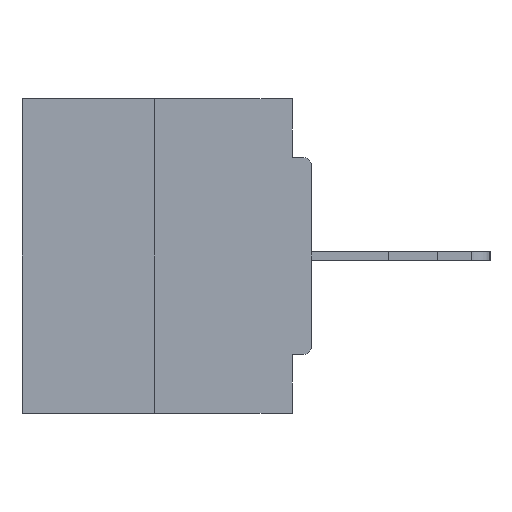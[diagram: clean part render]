
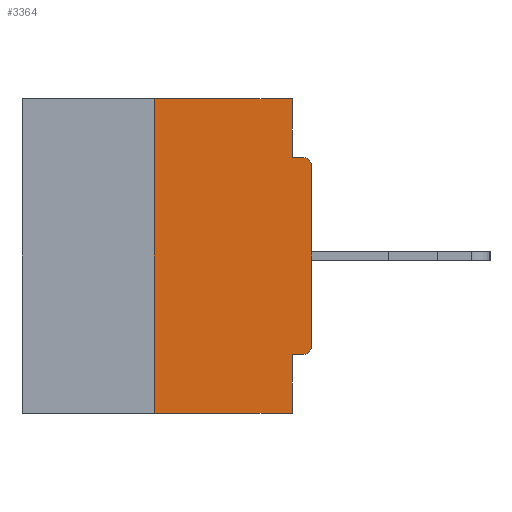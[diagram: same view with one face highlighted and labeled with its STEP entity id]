
A CAD part, left-side view. The second image highlights one B-rep face of the part: STEP entity #3364.
In plain terms, the highlighted planar face has unit normal (-1, 0, 0).
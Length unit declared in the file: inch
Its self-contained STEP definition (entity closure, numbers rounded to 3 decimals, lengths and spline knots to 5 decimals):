
#55 = FACE_OUTER_BOUND ( 'NONE', #7087, .T. ) ;
#73 = LINE ( 'NONE', #16672, #9234 ) ;
#126 = CARTESIAN_POINT ( 'NONE',  ( 0., 0.015, -0.0935 ) ) ;
#410 = CARTESIAN_POINT ( 'NONE',  ( 0., 0., -0.4065 ) ) ;
#1468 = EDGE_CURVE ( 'NONE', #32105, #14670, #10368, .T. ) ;
#2022 = CARTESIAN_POINT ( 'NONE',  ( 0., 0.015, -0.4065 ) ) ;
#3066 = EDGE_CURVE ( 'NONE', #25264, #31497, #32591, .T. ) ;
#3364 = ADVANCED_FACE ( 'NONE', ( #55 ), #19361, .F. ) ;
#3743 = LINE ( 'NONE', #22718, #32855 ) ;
#3805 = CIRCLE ( 'NONE', #9006, 0.015 ) ;
#3923 = CARTESIAN_POINT ( 'NONE',  ( 0., 0.25, 0. ) ) ;
#4043 = CARTESIAN_POINT ( 'NONE',  ( 0., 0.031, -0.4065 ) ) ;
#4228 = EDGE_CURVE ( 'NONE', #17173, #25264, #30328, .T. ) ;
#5555 = CARTESIAN_POINT ( 'NONE',  ( 0., 0.46, 0. ) ) ;
#5597 = EDGE_CURVE ( 'NONE', #6720, #14635, #3743, .T. ) ;
#5639 = CARTESIAN_POINT ( 'NONE',  ( 0., 0.031, -0.5 ) ) ;
#5778 = DIRECTION ( 'NONE',  ( -1., 0., 0. ) ) ;
#6102 = VECTOR ( 'NONE', #27866, 39.37008 ) ;
#6159 = DIRECTION ( 'NONE',  ( 0., 0., -1. ) ) ;
#6409 = EDGE_CURVE ( 'NONE', #32105, #17173, #73, .T. ) ;
#6720 = VERTEX_POINT ( 'NONE', #30334 ) ;
#7087 = EDGE_LOOP ( 'NONE', ( #32565, #34400, #19141, #24221, #24549, #12323, #35749, #17140, #16503, #34561 ) ) ;
#7121 = AXIS2_PLACEMENT_3D ( 'NONE', #14281, #5778, #6159 ) ;
#8180 = DIRECTION ( 'NONE',  ( -1., 0., 0. ) ) ;
#8782 = CARTESIAN_POINT ( 'NONE',  ( 0., 0., -0.0935 ) ) ;
#9006 = AXIS2_PLACEMENT_3D ( 'NONE', #16490, #8180, #11053 ) ;
#9234 = VECTOR ( 'NONE', #17524, 39.37008 ) ;
#10368 = LINE ( 'NONE', #29895, #19078 ) ;
#11053 = DIRECTION ( 'NONE',  ( 0., 0., -1. ) ) ;
#11419 = VECTOR ( 'NONE', #21452, 39.37008 ) ;
#11682 = DIRECTION ( 'NONE',  ( 0., 0., 1. ) ) ;
#12323 = ORIENTED_EDGE ( 'NONE', *, *, #14468, .T. ) ;
#12875 = CIRCLE ( 'NONE', #7121, 0.015 ) ;
#13216 = CARTESIAN_POINT ( 'NONE',  ( 0., 0.031, 0. ) ) ;
#14020 = LINE ( 'NONE', #8782, #33083 ) ;
#14063 = CARTESIAN_POINT ( 'NONE',  ( 0., 0.031, 0. ) ) ;
#14281 = CARTESIAN_POINT ( 'NONE',  ( 0., 0.015, -0.1085 ) ) ;
#14468 = EDGE_CURVE ( 'NONE', #30010, #6720, #3805, .T. ) ;
#14564 = EDGE_CURVE ( 'NONE', #19833, #14670, #30408, .T. ) ;
#14635 = VERTEX_POINT ( 'NONE', #25871 ) ;
#14670 = VERTEX_POINT ( 'NONE', #31123 ) ;
#15772 = EDGE_CURVE ( 'NONE', #31497, #31030, #14020, .T. ) ;
#16490 = CARTESIAN_POINT ( 'NONE',  ( 0., 0.015, -0.3915 ) ) ;
#16503 = ORIENTED_EDGE ( 'NONE', *, *, #15772, .F. ) ;
#16672 = CARTESIAN_POINT ( 'NONE',  ( 0., 0.25, 0. ) ) ;
#16907 = AXIS2_PLACEMENT_3D ( 'NONE', #30569, #19172, #24426 ) ;
#17140 = ORIENTED_EDGE ( 'NONE', *, *, #31890, .T. ) ;
#17173 = VERTEX_POINT ( 'NONE', #3923 ) ;
#17204 = CARTESIAN_POINT ( 'NONE',  ( 0., 0.031, -0.0935 ) ) ;
#17524 = DIRECTION ( 'NONE',  ( 0., 0., 1. ) ) ;
#18834 = DIRECTION ( 'NONE',  ( 0., 0., -1. ) ) ;
#19028 = DIRECTION ( 'NONE',  ( 0., -1., 0. ) ) ;
#19078 = VECTOR ( 'NONE', #19028, 39.37008 ) ;
#19141 = ORIENTED_EDGE ( 'NONE', *, *, #1468, .T. ) ;
#19172 = DIRECTION ( 'NONE',  ( 1., 0., 0. ) ) ;
#19361 = PLANE ( 'NONE',  #16907 ) ;
#19833 = VERTEX_POINT ( 'NONE', #4043 ) ;
#20471 = EDGE_CURVE ( 'NONE', #30010, #19833, #33476, .T. ) ;
#20882 = VECTOR ( 'NONE', #32403, 39.37008 ) ;
#21452 = DIRECTION ( 'NONE',  ( 0., -1., 0. ) ) ;
#22718 = CARTESIAN_POINT ( 'NONE',  ( 0., 0., 0. ) ) ;
#23989 = VECTOR ( 'NONE', #18834, 39.37008 ) ;
#24221 = ORIENTED_EDGE ( 'NONE', *, *, #14564, .F. ) ;
#24426 = DIRECTION ( 'NONE',  ( 0., 0., -1. ) ) ;
#24549 = ORIENTED_EDGE ( 'NONE', *, *, #20471, .F. ) ;
#25048 = DIRECTION ( 'NONE',  ( 0., -1., 0. ) ) ;
#25264 = VERTEX_POINT ( 'NONE', #14063 ) ;
#25871 = CARTESIAN_POINT ( 'NONE',  ( 0., 0., -0.1085 ) ) ;
#27866 = DIRECTION ( 'NONE',  ( 0., 1., 0. ) ) ;
#29895 = CARTESIAN_POINT ( 'NONE',  ( 0., 0.46, -0.5 ) ) ;
#30010 = VERTEX_POINT ( 'NONE', #2022 ) ;
#30328 = LINE ( 'NONE', #5555, #11419 ) ;
#30334 = CARTESIAN_POINT ( 'NONE',  ( 0., 0., -0.3915 ) ) ;
#30408 = LINE ( 'NONE', #5639, #23989 ) ;
#30569 = CARTESIAN_POINT ( 'NONE',  ( 0., 0.46, 0. ) ) ;
#31030 = VERTEX_POINT ( 'NONE', #126 ) ;
#31123 = CARTESIAN_POINT ( 'NONE',  ( 0., 0.031, -0.5 ) ) ;
#31497 = VERTEX_POINT ( 'NONE', #17204 ) ;
#31890 = EDGE_CURVE ( 'NONE', #14635, #31030, #12875, .T. ) ;
#32105 = VERTEX_POINT ( 'NONE', #33378 ) ;
#32403 = DIRECTION ( 'NONE',  ( 0., 0., -1. ) ) ;
#32565 = ORIENTED_EDGE ( 'NONE', *, *, #4228, .F. ) ;
#32591 = LINE ( 'NONE', #13216, #20882 ) ;
#32855 = VECTOR ( 'NONE', #11682, 39.37008 ) ;
#33083 = VECTOR ( 'NONE', #25048, 39.37008 ) ;
#33378 = CARTESIAN_POINT ( 'NONE',  ( 0., 0.25, -0.5 ) ) ;
#33476 = LINE ( 'NONE', #410, #6102 ) ;
#34400 = ORIENTED_EDGE ( 'NONE', *, *, #6409, .F. ) ;
#34561 = ORIENTED_EDGE ( 'NONE', *, *, #3066, .F. ) ;
#35749 = ORIENTED_EDGE ( 'NONE', *, *, #5597, .T. ) ;
